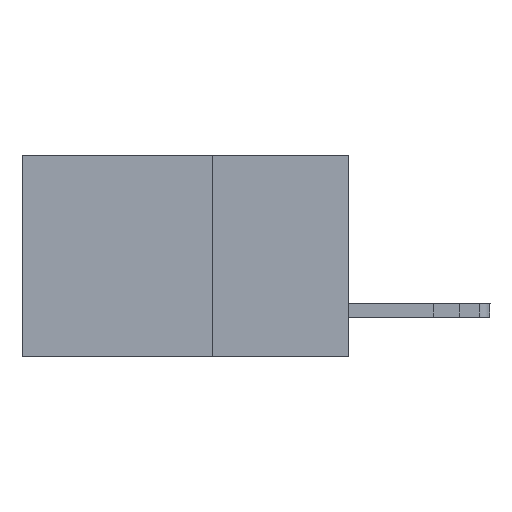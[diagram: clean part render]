
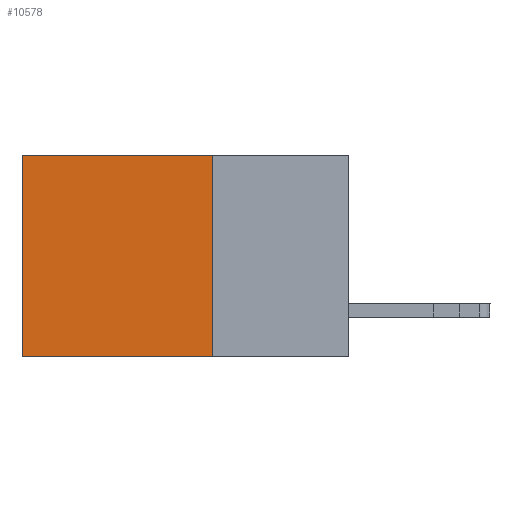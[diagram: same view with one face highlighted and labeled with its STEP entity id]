
A CAD part, left-side view. The second image highlights one B-rep face of the part: STEP entity #10578.
In plain terms, the highlighted planar face has unit normal (-1, 0, 0).
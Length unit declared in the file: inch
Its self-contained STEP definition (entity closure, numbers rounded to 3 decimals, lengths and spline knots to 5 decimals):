
#161 = AXIS2_PLACEMENT_3D ( 'NONE', #2379, #4579, #12329 ) ;
#345 = VERTEX_POINT ( 'NONE', #8672 ) ;
#1034 = LINE ( 'NONE', #10306, #4286 ) ;
#1486 = CARTESIAN_POINT ( 'NONE',  ( 0.2615, 0.25, -0.37 ) ) ;
#2379 = CARTESIAN_POINT ( 'NONE',  ( 0.2615, 0.25, -0.37 ) ) ;
#2534 = VERTEX_POINT ( 'NONE', #3971 ) ;
#2580 = FACE_OUTER_BOUND ( 'NONE', #3209, .T. ) ;
#3058 = CARTESIAN_POINT ( 'NONE',  ( 0.2615, 0.25, -0.37 ) ) ;
#3209 = EDGE_LOOP ( 'NONE', ( #6537, #5090, #10410, #12855 ) ) ;
#3291 = VERTEX_POINT ( 'NONE', #3058 ) ;
#3346 = EDGE_CURVE ( 'NONE', #7570, #2534, #4312, .T. ) ;
#3638 = VECTOR ( 'NONE', #8904, 39.37008 ) ;
#3663 = DIRECTION ( 'NONE',  ( 0., 1., 0. ) ) ;
#3971 = CARTESIAN_POINT ( 'NONE',  ( 0.2615, 0.6, -0.37 ) ) ;
#4160 = EDGE_CURVE ( 'NONE', #345, #7570, #1034, .T. ) ;
#4255 = VECTOR ( 'NONE', #10340, 39.37008 ) ;
#4286 = VECTOR ( 'NONE', #3663, 39.37008 ) ;
#4312 = LINE ( 'NONE', #14153, #9879 ) ;
#4537 = PLANE ( 'NONE',  #161 ) ;
#4579 = DIRECTION ( 'NONE',  ( 1., 0., 0. ) ) ;
#5090 = ORIENTED_EDGE ( 'NONE', *, *, #13715, .F. ) ;
#6537 = ORIENTED_EDGE ( 'NONE', *, *, #3346, .T. ) ;
#7570 = VERTEX_POINT ( 'NONE', #12913 ) ;
#7787 = CARTESIAN_POINT ( 'NONE',  ( 0.2615, 0.25, -0.37 ) ) ;
#8672 = CARTESIAN_POINT ( 'NONE',  ( 0.2615, 0.25, 0. ) ) ;
#8904 = DIRECTION ( 'NONE',  ( 0., 1., 0. ) ) ;
#9538 = LINE ( 'NONE', #7787, #3638 ) ;
#9790 = DIRECTION ( 'NONE',  ( 0., 0., -1. ) ) ;
#9879 = VECTOR ( 'NONE', #9790, 39.37008 ) ;
#10306 = CARTESIAN_POINT ( 'NONE',  ( 0.2615, 0.25, 0. ) ) ;
#10340 = DIRECTION ( 'NONE',  ( 0., 0., -1. ) ) ;
#10410 = ORIENTED_EDGE ( 'NONE', *, *, #11251, .F. ) ;
#10578 = ADVANCED_FACE ( 'NONE', ( #2580 ), #4537, .F. ) ;
#10872 = LINE ( 'NONE', #1486, #4255 ) ;
#11251 = EDGE_CURVE ( 'NONE', #345, #3291, #10872, .T. ) ;
#12329 = DIRECTION ( 'NONE',  ( 0., 0., -1. ) ) ;
#12855 = ORIENTED_EDGE ( 'NONE', *, *, #4160, .T. ) ;
#12913 = CARTESIAN_POINT ( 'NONE',  ( 0.2615, 0.6, 0. ) ) ;
#13715 = EDGE_CURVE ( 'NONE', #3291, #2534, #9538, .T. ) ;
#14153 = CARTESIAN_POINT ( 'NONE',  ( 0.2615, 0.6, -0.37 ) ) ;
